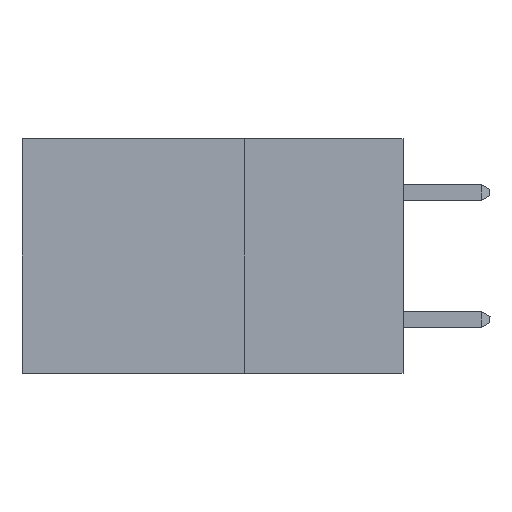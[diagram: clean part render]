
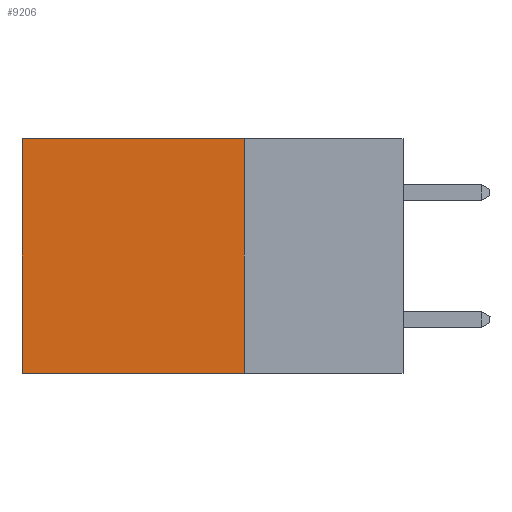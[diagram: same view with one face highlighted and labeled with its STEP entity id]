
A CAD part, left-side view. The second image highlights one B-rep face of the part: STEP entity #9206.
In plain terms, the highlighted planar face has unit normal (-1, 0, 0).
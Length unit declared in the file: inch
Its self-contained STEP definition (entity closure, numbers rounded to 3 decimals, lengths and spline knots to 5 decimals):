
#1052 = EDGE_CURVE ( 'NONE', #10931, #2399, #11599, .T. ) ;
#1079 = DIRECTION ( 'NONE',  ( 1., 0., 0. ) ) ;
#1627 = CARTESIAN_POINT ( 'NONE',  ( 0.2875, 0.6, -0.37 ) ) ;
#2399 = VERTEX_POINT ( 'NONE', #1627 ) ;
#3329 = CARTESIAN_POINT ( 'NONE',  ( 0.2875, 0.25, 0. ) ) ;
#5370 = CARTESIAN_POINT ( 'NONE',  ( 0.2875, 0.25, -0.37 ) ) ;
#5925 = VERTEX_POINT ( 'NONE', #3329 ) ;
#6834 = DIRECTION ( 'NONE',  ( 0., 0., -1. ) ) ;
#6893 = LINE ( 'NONE', #10213, #18357 ) ;
#6908 = VERTEX_POINT ( 'NONE', #19268 ) ;
#7111 = ORIENTED_EDGE ( 'NONE', *, *, #1052, .F. ) ;
#7414 = LINE ( 'NONE', #16486, #13519 ) ;
#9138 = LINE ( 'NONE', #17363, #16603 ) ;
#9171 = EDGE_CURVE ( 'NONE', #5925, #6908, #6893, .T. ) ;
#9206 = ADVANCED_FACE ( 'NONE', ( #18599 ), #14732, .F. ) ;
#9625 = ORIENTED_EDGE ( 'NONE', *, *, #12160, .T. ) ;
#10213 = CARTESIAN_POINT ( 'NONE',  ( 0.2875, 0.25, 0. ) ) ;
#10904 = DIRECTION ( 'NONE',  ( 0., 0., -1. ) ) ;
#10931 = VERTEX_POINT ( 'NONE', #5370 ) ;
#11599 = LINE ( 'NONE', #12988, #11849 ) ;
#11839 = ORIENTED_EDGE ( 'NONE', *, *, #9171, .T. ) ;
#11849 = VECTOR ( 'NONE', #17344, 39.37008 ) ;
#12160 = EDGE_CURVE ( 'NONE', #6908, #2399, #9138, .T. ) ;
#12988 = CARTESIAN_POINT ( 'NONE',  ( 0.2875, 0.25, -0.37 ) ) ;
#13519 = VECTOR ( 'NONE', #10904, 39.37008 ) ;
#14509 = AXIS2_PLACEMENT_3D ( 'NONE', #16158, #1079, #19028 ) ;
#14660 = DIRECTION ( 'NONE',  ( 0., 1., 0. ) ) ;
#14732 = PLANE ( 'NONE',  #14509 ) ;
#16158 = CARTESIAN_POINT ( 'NONE',  ( 0.2875, 0.25, 0. ) ) ;
#16486 = CARTESIAN_POINT ( 'NONE',  ( 0.2875, 0.25, 0. ) ) ;
#16603 = VECTOR ( 'NONE', #6834, 39.37008 ) ;
#16709 = EDGE_CURVE ( 'NONE', #5925, #10931, #7414, .T. ) ;
#17344 = DIRECTION ( 'NONE',  ( 0., 1., 0. ) ) ;
#17363 = CARTESIAN_POINT ( 'NONE',  ( 0.2875, 0.6, 0. ) ) ;
#17879 = ORIENTED_EDGE ( 'NONE', *, *, #16709, .F. ) ;
#18357 = VECTOR ( 'NONE', #14660, 39.37008 ) ;
#18498 = EDGE_LOOP ( 'NONE', ( #9625, #7111, #17879, #11839 ) ) ;
#18599 = FACE_OUTER_BOUND ( 'NONE', #18498, .T. ) ;
#19028 = DIRECTION ( 'NONE',  ( 0., 0., -1. ) ) ;
#19268 = CARTESIAN_POINT ( 'NONE',  ( 0.2875, 0.6, 0. ) ) ;
